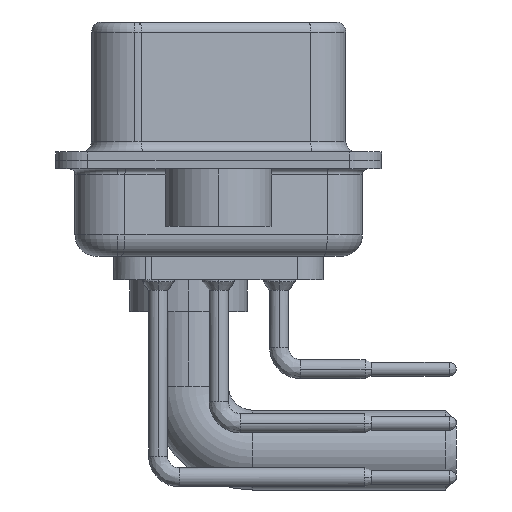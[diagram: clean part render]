
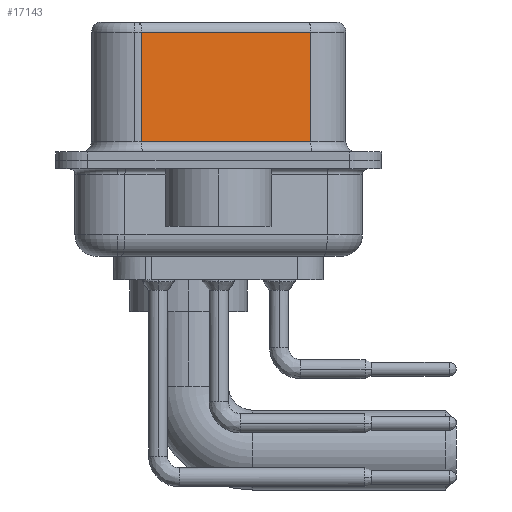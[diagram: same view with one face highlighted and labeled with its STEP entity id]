
A CAD part, left-side view. The second image highlights one B-rep face of the part: STEP entity #17143.
In plain terms, the highlighted planar face has unit normal (-0.985, -0.174, 0).
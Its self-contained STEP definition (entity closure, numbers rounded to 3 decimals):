
#1278 = ORIENTED_EDGE ( 'NONE', *, *, #8481, .F. ) ;
#2100 = VERTEX_POINT ( 'NONE', #2949 ) ;
#2471 = ORIENTED_EDGE ( 'NONE', *, *, #34340, .T. ) ;
#2584 = CARTESIAN_POINT ( 'NONE',  ( 5.132, -4.322, 0.9 ) ) ;
#2618 = ORIENTED_EDGE ( 'NONE', *, *, #23470, .T. ) ;
#2949 = CARTESIAN_POINT ( 'NONE',  ( 5.132, -4.322, 6.02 ) ) ;
#4276 = LINE ( 'NONE', #21668, #29928 ) ;
#5356 = CARTESIAN_POINT ( 'NONE',  ( 3.73, 3.628, 6.52 ) ) ;
#7654 = VECTOR ( 'NONE', #14990, 1000. ) ;
#8085 = CARTESIAN_POINT ( 'NONE',  ( 5.132, -4.322, 6.52 ) ) ;
#8481 = EDGE_CURVE ( 'NONE', #2100, #14084, #21682, .T. ) ;
#9717 = LINE ( 'NONE', #15191, #7654 ) ;
#11358 = CARTESIAN_POINT ( 'NONE',  ( 3.73, 3.628, 6.02 ) ) ;
#11472 = DIRECTION ( 'NONE',  ( 0.985, 0.174, 0. ) ) ;
#11875 = VECTOR ( 'NONE', #22767, 1000. ) ;
#12967 = CARTESIAN_POINT ( 'NONE',  ( 5.132, -4.322, 6.52 ) ) ;
#13672 = LINE ( 'NONE', #5356, #11875 ) ;
#14084 = VERTEX_POINT ( 'NONE', #2584 ) ;
#14288 = FACE_OUTER_BOUND ( 'NONE', #17591, .T. ) ;
#14990 = DIRECTION ( 'NONE',  ( -0.174, 0.985, 0. ) ) ;
#15191 = CARTESIAN_POINT ( 'NONE',  ( 5.132, -4.322, 6.02 ) ) ;
#17143 = ADVANCED_FACE ( 'NONE', ( #14288 ), #37416, .F. ) ;
#17396 = AXIS2_PLACEMENT_3D ( 'NONE', #8085, #11472, #23026 ) ;
#17591 = EDGE_LOOP ( 'NONE', ( #1278, #31482, #2471, #2618 ) ) ;
#19918 = VECTOR ( 'NONE', #33236, 1000. ) ;
#21668 = CARTESIAN_POINT ( 'NONE',  ( 5.132, -4.322, 0.9 ) ) ;
#21682 = LINE ( 'NONE', #12967, #19918 ) ;
#22767 = DIRECTION ( 'NONE',  ( 0., 0., -1. ) ) ;
#23026 = DIRECTION ( 'NONE',  ( -0.174, 0.985, 0. ) ) ;
#23470 = EDGE_CURVE ( 'NONE', #36338, #14084, #4276, .T. ) ;
#25013 = EDGE_CURVE ( 'NONE', #2100, #29384, #9717, .T. ) ;
#29384 = VERTEX_POINT ( 'NONE', #11358 ) ;
#29928 = VECTOR ( 'NONE', #33415, 1000. ) ;
#31482 = ORIENTED_EDGE ( 'NONE', *, *, #25013, .T. ) ;
#33236 = DIRECTION ( 'NONE',  ( 0., 0., -1. ) ) ;
#33415 = DIRECTION ( 'NONE',  ( 0.174, -0.985, 0. ) ) ;
#34340 = EDGE_CURVE ( 'NONE', #29384, #36338, #13672, .T. ) ;
#34822 = CARTESIAN_POINT ( 'NONE',  ( 3.73, 3.628, 0.9 ) ) ;
#36338 = VERTEX_POINT ( 'NONE', #34822 ) ;
#37416 = PLANE ( 'NONE',  #17396 ) ;
